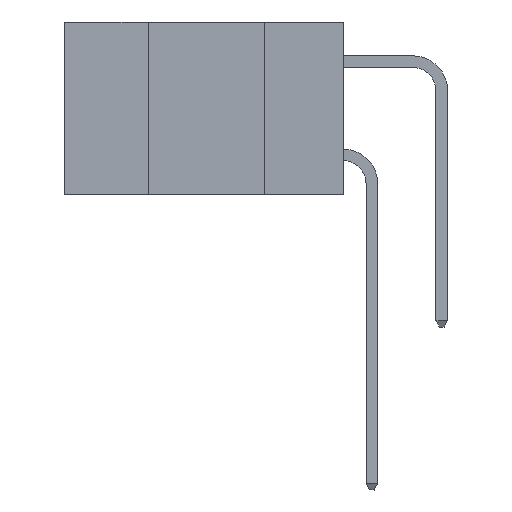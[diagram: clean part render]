
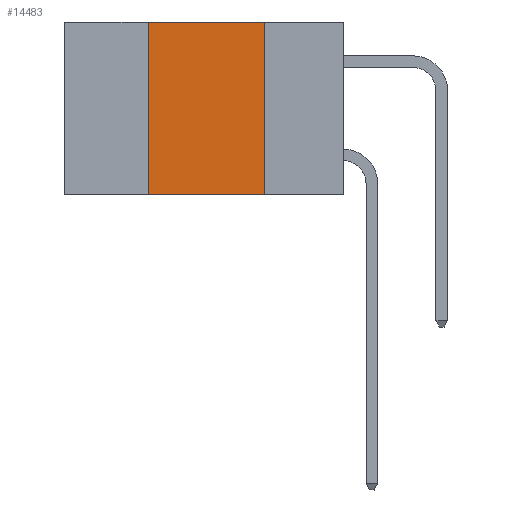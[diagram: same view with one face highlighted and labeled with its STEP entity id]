
A CAD part, left-side view. The second image highlights one B-rep face of the part: STEP entity #14483.
In plain terms, the highlighted planar face has unit normal (-1, 0, 0).
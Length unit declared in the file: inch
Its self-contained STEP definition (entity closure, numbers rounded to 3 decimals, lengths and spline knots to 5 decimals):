
#414 = ORIENTED_EDGE ( 'NONE', *, *, #3897, .F. ) ;
#1213 = VERTEX_POINT ( 'NONE', #12741 ) ;
#1285 = EDGE_LOOP ( 'NONE', ( #8332, #414, #5464, #9880 ) ) ;
#1832 = CARTESIAN_POINT ( 'NONE',  ( 0., 0.17, 0. ) ) ;
#1970 = CARTESIAN_POINT ( 'NONE',  ( 0., 0.42, -0.37 ) ) ;
#2100 = DIRECTION ( 'NONE',  ( 0., 0., 1. ) ) ;
#2605 = VERTEX_POINT ( 'NONE', #14564 ) ;
#2862 = VERTEX_POINT ( 'NONE', #1970 ) ;
#2992 = LINE ( 'NONE', #16588, #6903 ) ;
#3897 = EDGE_CURVE ( 'NONE', #19563, #1213, #2992, .T. ) ;
#5283 = CARTESIAN_POINT ( 'NONE',  ( 0., 0.6, 0. ) ) ;
#5464 = ORIENTED_EDGE ( 'NONE', *, *, #16933, .F. ) ;
#5620 = DIRECTION ( 'NONE',  ( 0., -1., 0. ) ) ;
#6509 = DIRECTION ( 'NONE',  ( 0., -1., 0. ) ) ;
#6903 = VECTOR ( 'NONE', #6509, 39.37008 ) ;
#6962 = DIRECTION ( 'NONE',  ( 0., 0., -1. ) ) ;
#8071 = LINE ( 'NONE', #12013, #13053 ) ;
#8332 = ORIENTED_EDGE ( 'NONE', *, *, #18005, .F. ) ;
#9719 = VECTOR ( 'NONE', #5620, 39.37008 ) ;
#9880 = ORIENTED_EDGE ( 'NONE', *, *, #15191, .T. ) ;
#10001 = FACE_OUTER_BOUND ( 'NONE', #1285, .T. ) ;
#10661 = CARTESIAN_POINT ( 'NONE',  ( 0., 0.42, 0. ) ) ;
#11930 = PLANE ( 'NONE',  #16530 ) ;
#12013 = CARTESIAN_POINT ( 'NONE',  ( 0., 0.42, 0. ) ) ;
#12741 = CARTESIAN_POINT ( 'NONE',  ( 0., 0.17, 0. ) ) ;
#13053 = VECTOR ( 'NONE', #2100, 39.37008 ) ;
#13534 = DIRECTION ( 'NONE',  ( 0., 0., -1. ) ) ;
#14201 = LINE ( 'NONE', #15649, #9719 ) ;
#14483 = ADVANCED_FACE ( 'NONE', ( #10001 ), #11930, .F. ) ;
#14564 = CARTESIAN_POINT ( 'NONE',  ( 0., 0.17, -0.37 ) ) ;
#15191 = EDGE_CURVE ( 'NONE', #2862, #2605, #14201, .T. ) ;
#15649 = CARTESIAN_POINT ( 'NONE',  ( 0., 0.6, -0.37 ) ) ;
#16530 = AXIS2_PLACEMENT_3D ( 'NONE', #5283, #16923, #6962 ) ;
#16588 = CARTESIAN_POINT ( 'NONE',  ( 0., 0.6, 0. ) ) ;
#16923 = DIRECTION ( 'NONE',  ( 1., 0., 0. ) ) ;
#16933 = EDGE_CURVE ( 'NONE', #2862, #19563, #8071, .T. ) ;
#18005 = EDGE_CURVE ( 'NONE', #1213, #2605, #21463, .T. ) ;
#19563 = VERTEX_POINT ( 'NONE', #10661 ) ;
#20944 = VECTOR ( 'NONE', #13534, 39.37008 ) ;
#21463 = LINE ( 'NONE', #1832, #20944 ) ;
